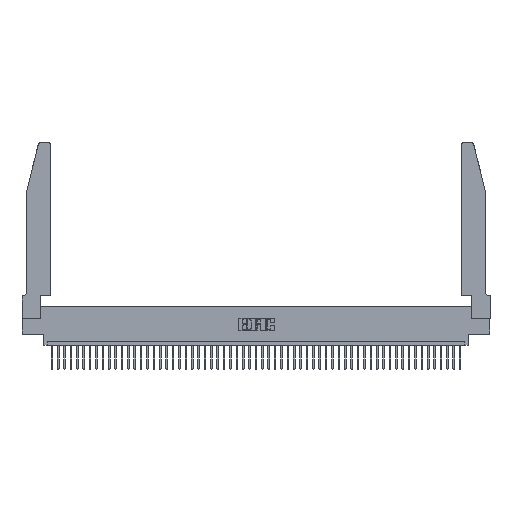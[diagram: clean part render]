
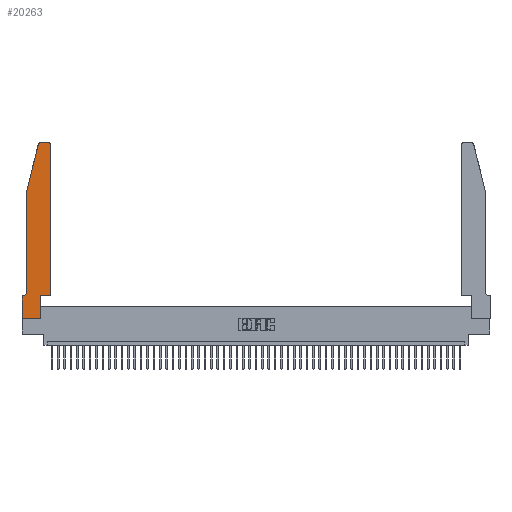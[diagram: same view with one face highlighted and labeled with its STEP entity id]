
A CAD part, top view. The second image highlights one B-rep face of the part: STEP entity #20263.
In plain terms, the highlighted planar face has unit normal (0, 0, 1).
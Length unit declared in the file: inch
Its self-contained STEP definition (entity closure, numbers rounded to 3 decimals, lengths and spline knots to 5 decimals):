
#459 = DIRECTION ( 'NONE',  ( 1., 0., 0. ) ) ;
#706 = EDGE_LOOP ( 'NONE', ( #3017, #39404, #4164, #45291, #49149, #41957, #37089, #30119, #42808, #4336, #33029, #29419 ) ) ;
#1992 = VERTEX_POINT ( 'NONE', #14226 ) ;
#2265 = DIRECTION ( 'NONE',  ( 0., -1., 0. ) ) ;
#2662 = AXIS2_PLACEMENT_3D ( 'NONE', #18027, #21982, #49356 ) ;
#3017 = ORIENTED_EDGE ( 'NONE', *, *, #15027, .T. ) ;
#3631 = VERTEX_POINT ( 'NONE', #26119 ) ;
#3850 = CARTESIAN_POINT ( 'NONE',  ( 0., 0., 0.37 ) ) ;
#3963 = VECTOR ( 'NONE', #6554, 39.37008 ) ;
#4164 = ORIENTED_EDGE ( 'NONE', *, *, #29628, .T. ) ;
#4336 = ORIENTED_EDGE ( 'NONE', *, *, #35178, .T. ) ;
#4582 = VERTEX_POINT ( 'NONE', #21841 ) ;
#5741 = FACE_OUTER_BOUND ( 'NONE', #706, .T. ) ;
#6114 = VECTOR ( 'NONE', #7380, 39.37008 ) ;
#6554 = DIRECTION ( 'NONE',  ( 1., 0., 0. ) ) ;
#7377 = LINE ( 'NONE', #17544, #37493 ) ;
#7380 = DIRECTION ( 'NONE',  ( 1., 0., 0. ) ) ;
#8082 = DIRECTION ( 'NONE',  ( 0., 0., -1. ) ) ;
#8732 = VECTOR ( 'NONE', #10609, 39.37008 ) ;
#8818 = CARTESIAN_POINT ( 'NONE',  ( 0.2865, 0.35, 0.37 ) ) ;
#9582 = VECTOR ( 'NONE', #23902, 39.37008 ) ;
#10085 = CARTESIAN_POINT ( 'NONE',  ( 0.2865, 0.35, 0.37 ) ) ;
#10609 = DIRECTION ( 'NONE',  ( -1., 0., 0. ) ) ;
#11489 = EDGE_CURVE ( 'NONE', #36728, #36637, #44785, .T. ) ;
#12090 = EDGE_CURVE ( 'NONE', #23364, #1992, #50145, .T. ) ;
#13946 = CARTESIAN_POINT ( 'NONE',  ( 0.4505, 0.35, 0.37 ) ) ;
#14226 = CARTESIAN_POINT ( 'NONE',  ( 0.25487, 2.72718, 0.37 ) ) ;
#14654 = CARTESIAN_POINT ( 'NONE',  ( 0.2865, 0., 0.37 ) ) ;
#15027 = EDGE_CURVE ( 'NONE', #23574, #23364, #29609, .T. ) ;
#16621 = VERTEX_POINT ( 'NONE', #18193 ) ;
#16700 = AXIS2_PLACEMENT_3D ( 'NONE', #23696, #8082, #35570 ) ;
#17459 = EDGE_CURVE ( 'NONE', #4582, #36728, #42775, .T. ) ;
#17544 = CARTESIAN_POINT ( 'NONE',  ( 0.0755, 0.35, 0.37 ) ) ;
#18027 = CARTESIAN_POINT ( 'NONE',  ( 0.284, 2.72, 0.37 ) ) ;
#18193 = CARTESIAN_POINT ( 'NONE',  ( 0.4505, 2.72, 0.37 ) ) ;
#18260 = CARTESIAN_POINT ( 'NONE',  ( 0.4205, 2.75, 0.37 ) ) ;
#19628 = CIRCLE ( 'NONE', #16700, 0.07 ) ;
#19784 = CARTESIAN_POINT ( 'NONE',  ( 0.4505, 0.35, 0.37 ) ) ;
#20263 = ADVANCED_FACE ( 'NONE', ( #5741 ), #24157, .T. ) ;
#21841 = CARTESIAN_POINT ( 'NONE',  ( 0., 0.35, 0.37 ) ) ;
#21982 = DIRECTION ( 'NONE',  ( 0., 0., 1. ) ) ;
#22023 = DIRECTION ( 'NONE',  ( -1., 0., 0. ) ) ;
#23338 = CIRCLE ( 'NONE', #39169, 0.03 ) ;
#23364 = VERTEX_POINT ( 'NONE', #24600 ) ;
#23574 = VERTEX_POINT ( 'NONE', #18260 ) ;
#23696 = CARTESIAN_POINT ( 'NONE',  ( 0.0055, 0.42, 0.37 ) ) ;
#23902 = DIRECTION ( 'NONE',  ( 0., 1., 0. ) ) ;
#24157 = PLANE ( 'NONE',  #32321 ) ;
#24190 = VERTEX_POINT ( 'NONE', #10085 ) ;
#24600 = CARTESIAN_POINT ( 'NONE',  ( 0.284, 2.75, 0.37 ) ) ;
#24774 = DIRECTION ( 'NONE',  ( 0., 1., 0. ) ) ;
#26119 = CARTESIAN_POINT ( 'NONE',  ( 0.0755, 2., 0.37 ) ) ;
#26239 = VECTOR ( 'NONE', #32547, 39.37008 ) ;
#27273 = LINE ( 'NONE', #29907, #3963 ) ;
#28059 = LINE ( 'NONE', #39896, #26239 ) ;
#28099 = DIRECTION ( 'NONE',  ( 0., 0., 1. ) ) ;
#28902 = CARTESIAN_POINT ( 'NONE',  ( 0.2605, 2.75, 0.37 ) ) ;
#29419 = ORIENTED_EDGE ( 'NONE', *, *, #38082, .T. ) ;
#29449 = DIRECTION ( 'NONE',  ( 0., 0., 1. ) ) ;
#29536 = CARTESIAN_POINT ( 'NONE',  ( 0.0755, 2., 0.37 ) ) ;
#29609 = LINE ( 'NONE', #28902, #8732 ) ;
#29628 = EDGE_CURVE ( 'NONE', #1992, #3631, #28059, .T. ) ;
#29907 = CARTESIAN_POINT ( 'NONE',  ( 0.4505, 0.35, 0.37 ) ) ;
#30119 = ORIENTED_EDGE ( 'NONE', *, *, #11489, .T. ) ;
#30796 = LINE ( 'NONE', #29536, #38768 ) ;
#30923 = CARTESIAN_POINT ( 'NONE',  ( 0., 0., 0.37 ) ) ;
#30957 = CARTESIAN_POINT ( 'NONE',  ( 0.0055, 0.35, 0.37 ) ) ;
#32092 = DIRECTION ( 'NONE',  ( 1., 0., 0. ) ) ;
#32321 = AXIS2_PLACEMENT_3D ( 'NONE', #48116, #28099, #32092 ) ;
#32547 = DIRECTION ( 'NONE',  ( -0.239, -0.971, 0. ) ) ;
#33029 = ORIENTED_EDGE ( 'NONE', *, *, #50465, .T. ) ;
#33993 = CARTESIAN_POINT ( 'NONE',  ( 0.0755, 0.42, 0.37 ) ) ;
#34772 = LINE ( 'NONE', #19784, #9582 ) ;
#35178 = EDGE_CURVE ( 'NONE', #24190, #47282, #27273, .T. ) ;
#35570 = DIRECTION ( 'NONE',  ( -1., 0., 0. ) ) ;
#35874 = DIRECTION ( 'NONE',  ( 0., -1., 0. ) ) ;
#36637 = VERTEX_POINT ( 'NONE', #14654 ) ;
#36728 = VERTEX_POINT ( 'NONE', #3850 ) ;
#37076 = EDGE_CURVE ( 'NONE', #3631, #42647, #30796, .T. ) ;
#37089 = ORIENTED_EDGE ( 'NONE', *, *, #17459, .T. ) ;
#37493 = VECTOR ( 'NONE', #22023, 39.37008 ) ;
#38082 = EDGE_CURVE ( 'NONE', #16621, #23574, #23338, .T. ) ;
#38768 = VECTOR ( 'NONE', #2265, 39.37008 ) ;
#38890 = CARTESIAN_POINT ( 'NONE',  ( 0.4205, 2.72, 0.37 ) ) ;
#39169 = AXIS2_PLACEMENT_3D ( 'NONE', #38890, #29449, #459 ) ;
#39404 = ORIENTED_EDGE ( 'NONE', *, *, #12090, .T. ) ;
#39896 = CARTESIAN_POINT ( 'NONE',  ( 0.0755, 2., 0.37 ) ) ;
#41957 = ORIENTED_EDGE ( 'NONE', *, *, #45415, .T. ) ;
#42647 = VERTEX_POINT ( 'NONE', #33993 ) ;
#42775 = LINE ( 'NONE', #47784, #50096 ) ;
#42808 = ORIENTED_EDGE ( 'NONE', *, *, #47118, .T. ) ;
#44785 = LINE ( 'NONE', #30923, #6114 ) ;
#44945 = VERTEX_POINT ( 'NONE', #30957 ) ;
#45291 = ORIENTED_EDGE ( 'NONE', *, *, #37076, .T. ) ;
#45415 = EDGE_CURVE ( 'NONE', #44945, #4582, #7377, .T. ) ;
#45728 = EDGE_CURVE ( 'NONE', #42647, #44945, #19628, .T. ) ;
#47118 = EDGE_CURVE ( 'NONE', #36637, #24190, #49191, .T. ) ;
#47282 = VERTEX_POINT ( 'NONE', #13946 ) ;
#47784 = CARTESIAN_POINT ( 'NONE',  ( 0., 0., 0.37 ) ) ;
#48116 = CARTESIAN_POINT ( 'NONE',  ( 0., 0.35, 0.37 ) ) ;
#49149 = ORIENTED_EDGE ( 'NONE', *, *, #45728, .T. ) ;
#49191 = LINE ( 'NONE', #8818, #50409 ) ;
#49356 = DIRECTION ( 'NONE',  ( 1., 0., 0. ) ) ;
#50096 = VECTOR ( 'NONE', #35874, 39.37008 ) ;
#50145 = CIRCLE ( 'NONE', #2662, 0.03 ) ;
#50409 = VECTOR ( 'NONE', #24774, 39.37008 ) ;
#50465 = EDGE_CURVE ( 'NONE', #47282, #16621, #34772, .T. ) ;
